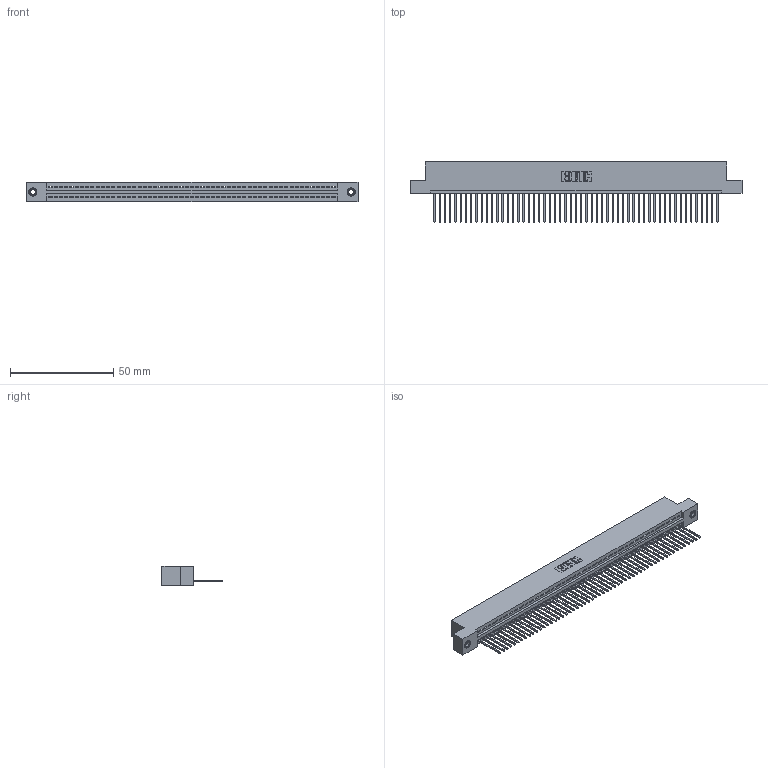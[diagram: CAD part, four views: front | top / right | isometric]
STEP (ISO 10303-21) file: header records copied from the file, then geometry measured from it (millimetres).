
FILE_DESCRIPTION (( 'STEP AP203' ), '1' );
FILE_NAME ('395-055-540-108.STEP', '2018-11-21T23:23:41', ( '' ), ( '' ), 'SwSTEP 2.0', 'SolidWorks 2016', '' );
FILE_SCHEMA (( 'CONFIG_CONTROL_DESIGN' ));
Length unit declared in the file: inch
Products named in the file (4): 345 Part_Flush Mounting Lugs - 0.156 Dia-TI; 345-250-001_345-250-003-102; 395-055-540-108; 345-292-001_345-293-140
Assembly tree (58 placements, depth 2):
  395-055-540-108
    345 Part_Flush Mounting Lugs - 0.156 Dia-TI
    345-292-001_345-293-140  x55
    345-250-001_345-250-003-102  x2
Bounding box: 160.91 x 29.13 x 9.4 mm (x, y, z)
Volume: 15457.8 mm3; surface area: 21273.7 mm2
Topology: 58 solids, 58 shells, 3376 faces, 10157 edges, 6690 vertices
Faces by surface type: plane 2312, cylinder 1048, cone 12, torus 4
Entity records: 40848 total; most frequent: CARTESIAN_POINT 7056, ORIENTED_EDGE 7038, DIRECTION 6171, EDGE_CURVE 3519, LINE 3147, VECTOR 3147, VERTEX_POINT 2340, AXIS2_PLACEMENT_3D 1512
